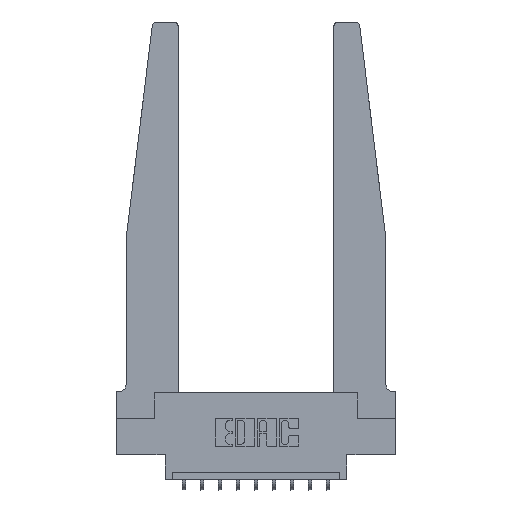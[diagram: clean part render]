
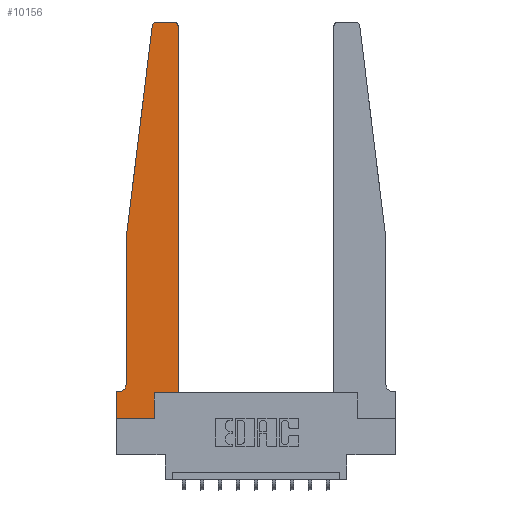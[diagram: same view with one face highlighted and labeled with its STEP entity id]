
A CAD part, top view. The second image highlights one B-rep face of the part: STEP entity #10156.
In plain terms, the highlighted planar face has unit normal (0, 0, 1).
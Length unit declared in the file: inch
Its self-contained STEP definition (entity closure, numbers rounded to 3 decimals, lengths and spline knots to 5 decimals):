
#207 = EDGE_CURVE ( 'NONE', #11003, #4898, #14061, .T. ) ;
#232 = LINE ( 'NONE', #10676, #605 ) ;
#367 = LINE ( 'NONE', #13716, #3131 ) ;
#605 = VECTOR ( 'NONE', #2556, 39.37008 ) ;
#761 = ORIENTED_EDGE ( 'NONE', *, *, #207, .T. ) ;
#833 = EDGE_CURVE ( 'NONE', #10415, #12798, #232, .T. ) ;
#1076 = CARTESIAN_POINT ( 'NONE',  ( 0.015, 0.2375, 0.37 ) ) ;
#1077 = ORIENTED_EDGE ( 'NONE', *, *, #13073, .T. ) ;
#1193 = CARTESIAN_POINT ( 'NONE',  ( 0.27653, 2.72, 0.37 ) ) ;
#1286 = VERTEX_POINT ( 'NONE', #7930 ) ;
#1546 = CARTESIAN_POINT ( 'NONE',  ( 0.065, 0.2375, 0.37 ) ) ;
#1732 = VECTOR ( 'NONE', #14891, 39.37008 ) ;
#1907 = ORIENTED_EDGE ( 'NONE', *, *, #833, .T. ) ;
#1956 = CARTESIAN_POINT ( 'NONE',  ( 0., 0., 0.37 ) ) ;
#2037 = ORIENTED_EDGE ( 'NONE', *, *, #2198, .T. ) ;
#2061 = AXIS2_PLACEMENT_3D ( 'NONE', #1193, #9350, #2386 ) ;
#2198 = EDGE_CURVE ( 'NONE', #4898, #11039, #4424, .T. ) ;
#2248 = LINE ( 'NONE', #9164, #4983 ) ;
#2266 = DIRECTION ( 'NONE',  ( -1., 0., 0. ) ) ;
#2383 = VECTOR ( 'NONE', #11686, 39.37008 ) ;
#2386 = DIRECTION ( 'NONE',  ( 1., 0., 0. ) ) ;
#2541 = EDGE_CURVE ( 'NONE', #9108, #5464, #367, .T. ) ;
#2556 = DIRECTION ( 'NONE',  ( -1., 0., 0. ) ) ;
#2791 = CARTESIAN_POINT ( 'NONE',  ( 0.425, 0.18, 0.37 ) ) ;
#2911 = CARTESIAN_POINT ( 'NONE',  ( 0., 0.1875, 0.37 ) ) ;
#3103 = PLANE ( 'NONE',  #8133 ) ;
#3131 = VECTOR ( 'NONE', #5723, 39.37008 ) ;
#3503 = EDGE_CURVE ( 'NONE', #12798, #9510, #14644, .T. ) ;
#3544 = CARTESIAN_POINT ( 'NONE',  ( 0., 0., 0.37 ) ) ;
#3624 = ORIENTED_EDGE ( 'NONE', *, *, #3832, .T. ) ;
#3820 = CARTESIAN_POINT ( 'NONE',  ( 0., 0., 0.37 ) ) ;
#3827 = CARTESIAN_POINT ( 'NONE',  ( 0.24675, 2.72367, 0.37 ) ) ;
#3832 = EDGE_CURVE ( 'NONE', #9510, #1286, #10006, .T. ) ;
#3900 = ORIENTED_EDGE ( 'NONE', *, *, #11905, .T. ) ;
#3960 = VERTEX_POINT ( 'NONE', #7968 ) ;
#4163 = ORIENTED_EDGE ( 'NONE', *, *, #2541, .T. ) ;
#4191 = CARTESIAN_POINT ( 'NONE',  ( 0.395, 2.72, 0.37 ) ) ;
#4279 = DIRECTION ( 'NONE',  ( 1., 0., 0. ) ) ;
#4303 = DIRECTION ( 'NONE',  ( 1., 0., 0. ) ) ;
#4335 = ORIENTED_EDGE ( 'NONE', *, *, #13440, .T. ) ;
#4424 = LINE ( 'NONE', #8462, #10241 ) ;
#4853 = CIRCLE ( 'NONE', #9906, 0.05 ) ;
#4898 = VERTEX_POINT ( 'NONE', #4996 ) ;
#4983 = VECTOR ( 'NONE', #14906, 39.37008 ) ;
#4996 = CARTESIAN_POINT ( 'NONE',  ( 0.065, 1.25, 0.37 ) ) ;
#5288 = CIRCLE ( 'NONE', #2061, 0.03 ) ;
#5380 = DIRECTION ( 'NONE',  ( 1., 0., 0. ) ) ;
#5464 = VERTEX_POINT ( 'NONE', #13061 ) ;
#5723 = DIRECTION ( 'NONE',  ( -1., 0., 0. ) ) ;
#6329 = CARTESIAN_POINT ( 'NONE',  ( 0.2605, 0.18, 0.37 ) ) ;
#6608 = CARTESIAN_POINT ( 'NONE',  ( 0.425, 0.18, 0.37 ) ) ;
#6939 = VECTOR ( 'NONE', #4303, 39.37008 ) ;
#7792 = VECTOR ( 'NONE', #12915, 39.37008 ) ;
#7930 = CARTESIAN_POINT ( 'NONE',  ( 0.2605, 0., 0.37 ) ) ;
#7968 = CARTESIAN_POINT ( 'NONE',  ( 0.425, 2.72, 0.37 ) ) ;
#8133 = AXIS2_PLACEMENT_3D ( 'NONE', #13480, #11237, #4279 ) ;
#8141 = EDGE_CURVE ( 'NONE', #5464, #11003, #5288, .T. ) ;
#8462 = CARTESIAN_POINT ( 'NONE',  ( 0.065, 1.25, 0.37 ) ) ;
#8826 = AXIS2_PLACEMENT_3D ( 'NONE', #4191, #12335, #5380 ) ;
#8951 = CARTESIAN_POINT ( 'NONE',  ( 0.395, 2.75, 0.37 ) ) ;
#9108 = VERTEX_POINT ( 'NONE', #8951 ) ;
#9164 = CARTESIAN_POINT ( 'NONE',  ( 0.425, 0.18, 0.37 ) ) ;
#9246 = DIRECTION ( 'NONE',  ( 0., 0., -1. ) ) ;
#9350 = DIRECTION ( 'NONE',  ( 0., 0., 1. ) ) ;
#9412 = EDGE_CURVE ( 'NONE', #1286, #10046, #13902, .T. ) ;
#9418 = CARTESIAN_POINT ( 'NONE',  ( 0.015, 0.1875, 0.37 ) ) ;
#9510 = VERTEX_POINT ( 'NONE', #3820 ) ;
#9626 = DIRECTION ( 'NONE',  ( 0., -1., 0. ) ) ;
#9886 = ORIENTED_EDGE ( 'NONE', *, *, #3503, .T. ) ;
#9906 = AXIS2_PLACEMENT_3D ( 'NONE', #1076, #9246, #2266 ) ;
#10006 = LINE ( 'NONE', #1956, #6939 ) ;
#10046 = VERTEX_POINT ( 'NONE', #6329 ) ;
#10156 = ADVANCED_FACE ( 'NONE', ( #11033 ), #3103, .T. ) ;
#10241 = VECTOR ( 'NONE', #9626, 39.37008 ) ;
#10415 = VERTEX_POINT ( 'NONE', #9418 ) ;
#10634 = VERTEX_POINT ( 'NONE', #2791 ) ;
#10650 = VECTOR ( 'NONE', #13505, 39.37008 ) ;
#10676 = CARTESIAN_POINT ( 'NONE',  ( 0.065, 0.1875, 0.37 ) ) ;
#11003 = VERTEX_POINT ( 'NONE', #3827 ) ;
#11033 = FACE_OUTER_BOUND ( 'NONE', #15007, .T. ) ;
#11039 = VERTEX_POINT ( 'NONE', #1546 ) ;
#11192 = EDGE_CURVE ( 'NONE', #3960, #9108, #13329, .T. ) ;
#11237 = DIRECTION ( 'NONE',  ( 0., 0., 1. ) ) ;
#11477 = ORIENTED_EDGE ( 'NONE', *, *, #9412, .T. ) ;
#11686 = DIRECTION ( 'NONE',  ( 0., -1., 0. ) ) ;
#11905 = EDGE_CURVE ( 'NONE', #10046, #10634, #13681, .T. ) ;
#12335 = DIRECTION ( 'NONE',  ( 0., 0., 1. ) ) ;
#12798 = VERTEX_POINT ( 'NONE', #2911 ) ;
#12892 = ORIENTED_EDGE ( 'NONE', *, *, #11192, .T. ) ;
#12915 = DIRECTION ( 'NONE',  ( 0., 1., 0. ) ) ;
#13061 = CARTESIAN_POINT ( 'NONE',  ( 0.27653, 2.75, 0.37 ) ) ;
#13073 = EDGE_CURVE ( 'NONE', #10634, #3960, #2248, .T. ) ;
#13222 = ORIENTED_EDGE ( 'NONE', *, *, #8141, .T. ) ;
#13329 = CIRCLE ( 'NONE', #8826, 0.03 ) ;
#13440 = EDGE_CURVE ( 'NONE', #11039, #10415, #4853, .T. ) ;
#13480 = CARTESIAN_POINT ( 'NONE',  ( 0., 0.1875, 0.37 ) ) ;
#13505 = DIRECTION ( 'NONE',  ( 1., 0., 0. ) ) ;
#13681 = LINE ( 'NONE', #6608, #10650 ) ;
#13716 = CARTESIAN_POINT ( 'NONE',  ( 0.25, 2.75, 0.37 ) ) ;
#13893 = CARTESIAN_POINT ( 'NONE',  ( 0.065, 1.25, 0.37 ) ) ;
#13902 = LINE ( 'NONE', #14060, #7792 ) ;
#14060 = CARTESIAN_POINT ( 'NONE',  ( 0.2605, 0.18, 0.37 ) ) ;
#14061 = LINE ( 'NONE', #13893, #1732 ) ;
#14644 = LINE ( 'NONE', #3544, #2383 ) ;
#14891 = DIRECTION ( 'NONE',  ( -0.122, -0.992, 0. ) ) ;
#14906 = DIRECTION ( 'NONE',  ( 0., 1., 0. ) ) ;
#15007 = EDGE_LOOP ( 'NONE', ( #4163, #13222, #761, #2037, #4335, #1907, #9886, #3624, #11477, #3900, #1077, #12892 ) ) ;
